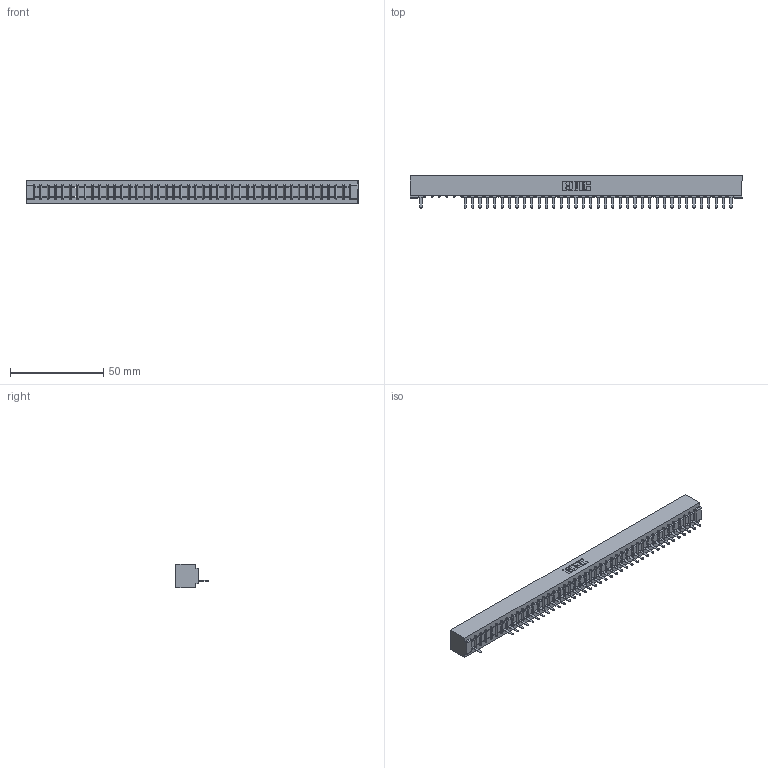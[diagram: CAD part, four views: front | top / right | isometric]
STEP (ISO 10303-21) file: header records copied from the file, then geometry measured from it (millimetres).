
FILE_DESCRIPTION (( 'STEP AP203' ), '1' );
FILE_NAME ('357-043-521-101.STEP', '2018-08-11T10:12:10', ( '' ), ( '' ), 'SwSTEP 2.0', 'SolidWorks 2016', '' );
FILE_SCHEMA (( 'CONFIG_CONTROL_DESIGN' ));
Length unit declared in the file: inch
Products named in the file (3): 307 Part_No Mounting Lugs; 307-290-002_521; 357-043-521-101
Assembly tree (39 placements, depth 2):
  357-043-521-101
    307 Part_No Mounting Lugs
    307-290-002_521  x38
Bounding box: 178.26 x 17.42 x 12.7 mm (x, y, z)
Volume: 19498.5 mm3; surface area: 23967.7 mm2
Topology: 39 solids, 39 shells, 3066 faces, 9435 edges, 6170 vertices
Faces by surface type: plane 1836, cylinder 1142, sphere 88
Entity records: 37020 total; most frequent: CARTESIAN_POINT 6267, ORIENTED_EDGE 6262, DIRECTION 6081, EDGE_CURVE 3131, LINE 2401, VECTOR 2401, VERTEX_POINT 2026, AXIS2_PLACEMENT_3D 1840
